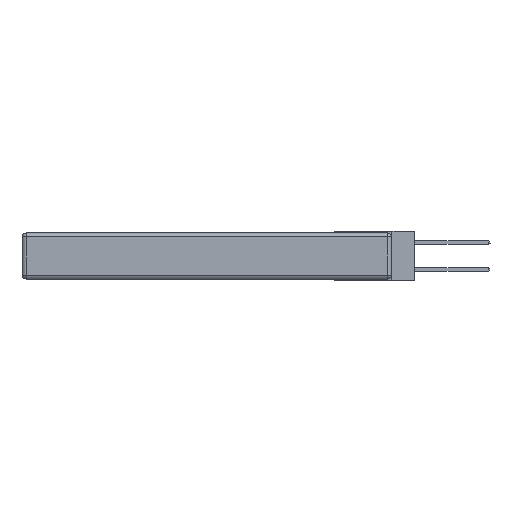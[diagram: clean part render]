
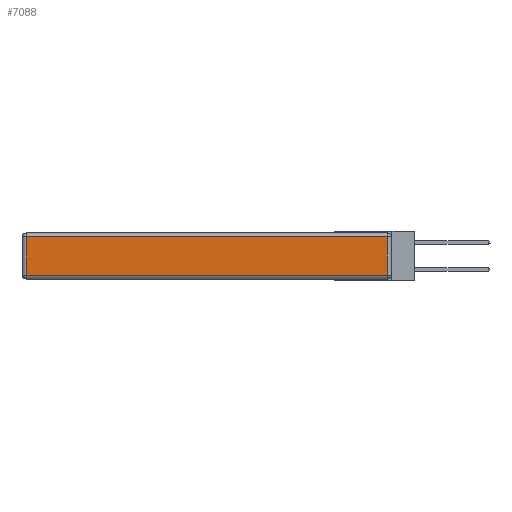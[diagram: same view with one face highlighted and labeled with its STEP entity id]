
A CAD part, left-side view. The second image highlights one B-rep face of the part: STEP entity #7088.
In plain terms, the highlighted planar face has unit normal (-1, 0, 0).
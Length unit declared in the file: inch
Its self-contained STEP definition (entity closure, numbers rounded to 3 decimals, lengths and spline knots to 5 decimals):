
#583 = DIRECTION ( 'NONE',  ( -1., 0., 0. ) ) ;
#2352 = DIRECTION ( 'NONE',  ( 0., -1., 0. ) ) ;
#3250 = EDGE_CURVE ( 'NONE', #6986, #18329, #8469, .T. ) ;
#3330 = LINE ( 'NONE', #23714, #25426 ) ;
#3397 = CARTESIAN_POINT ( 'NONE',  ( 0., 2.72, -0.03 ) ) ;
#3471 = DIRECTION ( 'NONE',  ( 0., 0., 1. ) ) ;
#3814 = EDGE_LOOP ( 'NONE', ( #20086, #3852, #17625, #25882 ) ) ;
#3852 = ORIENTED_EDGE ( 'NONE', *, *, #3250, .T. ) ;
#6777 = CARTESIAN_POINT ( 'NONE',  ( 0., 0.03, -0.343 ) ) ;
#6986 = VERTEX_POINT ( 'NONE', #11001 ) ;
#7088 = ADVANCED_FACE ( 'NONE', ( #20730 ), #13421, .T. ) ;
#7583 = EDGE_CURVE ( 'NONE', #13644, #24923, #21042, .T. ) ;
#8469 = LINE ( 'NONE', #6777, #16207 ) ;
#10613 = DIRECTION ( 'NONE',  ( 0., 0., -1. ) ) ;
#11001 = CARTESIAN_POINT ( 'NONE',  ( 0., 0.03, -0.313 ) ) ;
#12759 = LINE ( 'NONE', #12910, #18769 ) ;
#12910 = CARTESIAN_POINT ( 'NONE',  ( 0., 0., -0.313 ) ) ;
#13421 = PLANE ( 'NONE',  #25964 ) ;
#13644 = VERTEX_POINT ( 'NONE', #3397 ) ;
#14987 = CARTESIAN_POINT ( 'NONE',  ( 0., 2.72, -0.343 ) ) ;
#16207 = VECTOR ( 'NONE', #21739, 39.37008 ) ;
#16294 = CARTESIAN_POINT ( 'NONE',  ( 0., 2.72, -0.313 ) ) ;
#16404 = CARTESIAN_POINT ( 'NONE',  ( 0., 0.03, -0.03 ) ) ;
#16965 = EDGE_CURVE ( 'NONE', #18329, #13644, #3330, .T. ) ;
#17625 = ORIENTED_EDGE ( 'NONE', *, *, #16965, .T. ) ;
#18329 = VERTEX_POINT ( 'NONE', #16404 ) ;
#18769 = VECTOR ( 'NONE', #2352, 39.37008 ) ;
#19043 = VECTOR ( 'NONE', #10613, 39.37008 ) ;
#19336 = EDGE_CURVE ( 'NONE', #24923, #6986, #12759, .T. ) ;
#19511 = DIRECTION ( 'NONE',  ( 0., 1., 0. ) ) ;
#20086 = ORIENTED_EDGE ( 'NONE', *, *, #19336, .T. ) ;
#20097 = CARTESIAN_POINT ( 'NONE',  ( 0., 0., -0.343 ) ) ;
#20730 = FACE_OUTER_BOUND ( 'NONE', #3814, .T. ) ;
#21042 = LINE ( 'NONE', #14987, #19043 ) ;
#21739 = DIRECTION ( 'NONE',  ( 0., 0., 1. ) ) ;
#23714 = CARTESIAN_POINT ( 'NONE',  ( 0., 2.75, -0.03 ) ) ;
#24923 = VERTEX_POINT ( 'NONE', #16294 ) ;
#25426 = VECTOR ( 'NONE', #19511, 39.37008 ) ;
#25882 = ORIENTED_EDGE ( 'NONE', *, *, #7583, .T. ) ;
#25964 = AXIS2_PLACEMENT_3D ( 'NONE', #20097, #583, #3471 ) ;
